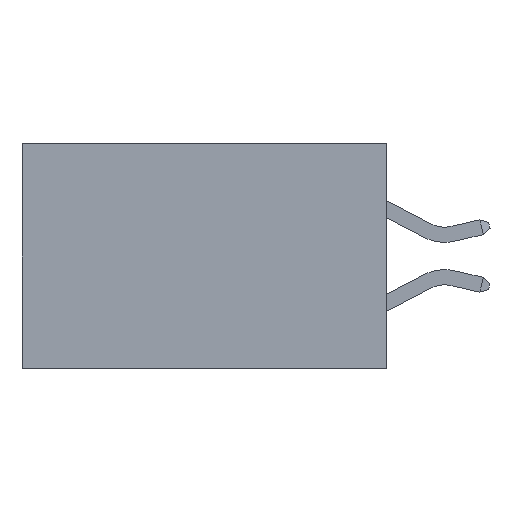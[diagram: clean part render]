
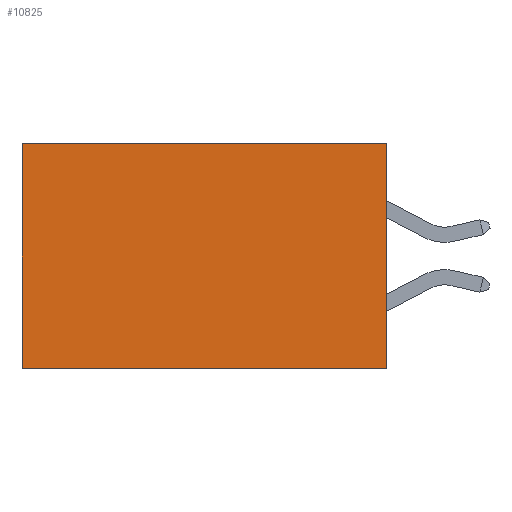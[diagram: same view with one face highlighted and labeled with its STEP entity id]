
A CAD part, left-side view. The second image highlights one B-rep face of the part: STEP entity #10825.
In plain terms, the highlighted planar face has unit normal (-1, 0, 0).
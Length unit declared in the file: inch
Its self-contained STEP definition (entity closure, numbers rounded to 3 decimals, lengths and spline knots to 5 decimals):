
#1164 = EDGE_CURVE ( 'NONE', #21208, #3631, #20284, .T. ) ;
#2301 = PLANE ( 'NONE',  #17880 ) ;
#3631 = VERTEX_POINT ( 'NONE', #10499 ) ;
#5949 = CARTESIAN_POINT ( 'NONE',  ( 0.2615, 0., -0.37 ) ) ;
#6599 = VECTOR ( 'NONE', #25126, 39.37008 ) ;
#6687 = VERTEX_POINT ( 'NONE', #20137 ) ;
#7086 = VERTEX_POINT ( 'NONE', #13150 ) ;
#7375 = CARTESIAN_POINT ( 'NONE',  ( 0.2615, 0., 0. ) ) ;
#7732 = VECTOR ( 'NONE', #23443, 39.37008 ) ;
#9255 = DIRECTION ( 'NONE',  ( 0., 0., -1. ) ) ;
#10499 = CARTESIAN_POINT ( 'NONE',  ( 0.2615, 0.6, -0.37 ) ) ;
#10732 = FACE_OUTER_BOUND ( 'NONE', #19460, .T. ) ;
#10825 = ADVANCED_FACE ( 'NONE', ( #10732 ), #2301, .F. ) ;
#11749 = LINE ( 'NONE', #25804, #17236 ) ;
#13150 = CARTESIAN_POINT ( 'NONE',  ( 0.2615, 0., 0. ) ) ;
#14627 = EDGE_CURVE ( 'NONE', #7086, #6687, #15249, .T. ) ;
#15249 = LINE ( 'NONE', #7375, #6599 ) ;
#17236 = VECTOR ( 'NONE', #9255, 39.37008 ) ;
#17393 = LINE ( 'NONE', #18973, #7732 ) ;
#17446 = EDGE_CURVE ( 'NONE', #7086, #21208, #17393, .T. ) ;
#17614 = ORIENTED_EDGE ( 'NONE', *, *, #17446, .F. ) ;
#17676 = CARTESIAN_POINT ( 'NONE',  ( 0.2615, 0., -0.37 ) ) ;
#17880 = AXIS2_PLACEMENT_3D ( 'NONE', #18344, #18728, #22421 ) ;
#18306 = DIRECTION ( 'NONE',  ( 0., 1., 0. ) ) ;
#18344 = CARTESIAN_POINT ( 'NONE',  ( 0.2615, 0., -0.37 ) ) ;
#18537 = ORIENTED_EDGE ( 'NONE', *, *, #1164, .F. ) ;
#18728 = DIRECTION ( 'NONE',  ( 1., 0., 0. ) ) ;
#18973 = CARTESIAN_POINT ( 'NONE',  ( 0.2615, 0., -0.37 ) ) ;
#19460 = EDGE_LOOP ( 'NONE', ( #25773, #18537, #17614, #23077 ) ) ;
#20137 = CARTESIAN_POINT ( 'NONE',  ( 0.2615, 0.6, 0. ) ) ;
#20284 = LINE ( 'NONE', #5949, #21149 ) ;
#21149 = VECTOR ( 'NONE', #18306, 39.37008 ) ;
#21208 = VERTEX_POINT ( 'NONE', #17676 ) ;
#22421 = DIRECTION ( 'NONE',  ( 0., 0., -1. ) ) ;
#23019 = EDGE_CURVE ( 'NONE', #6687, #3631, #11749, .T. ) ;
#23077 = ORIENTED_EDGE ( 'NONE', *, *, #14627, .T. ) ;
#23443 = DIRECTION ( 'NONE',  ( 0., 0., -1. ) ) ;
#25126 = DIRECTION ( 'NONE',  ( 0., 1., 0. ) ) ;
#25773 = ORIENTED_EDGE ( 'NONE', *, *, #23019, .T. ) ;
#25804 = CARTESIAN_POINT ( 'NONE',  ( 0.2615, 0.6, -0.37 ) ) ;
